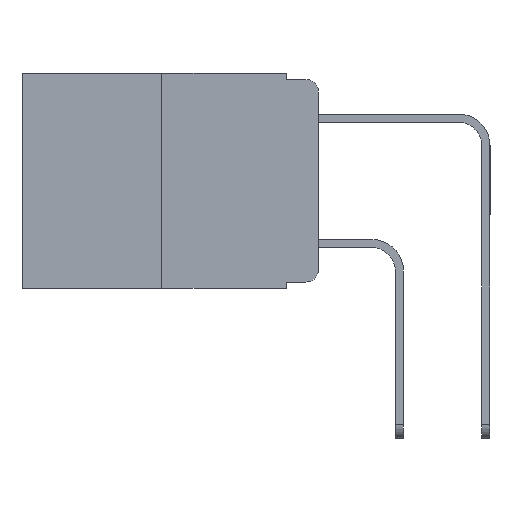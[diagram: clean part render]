
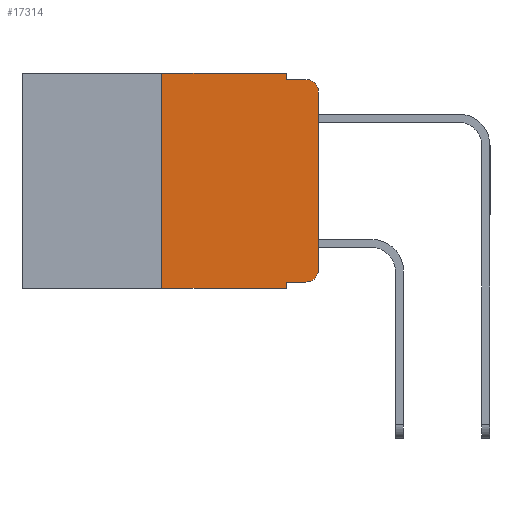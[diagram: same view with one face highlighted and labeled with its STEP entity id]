
A CAD part, left-side view. The second image highlights one B-rep face of the part: STEP entity #17314.
In plain terms, the highlighted planar face has unit normal (-1, 0, 0).
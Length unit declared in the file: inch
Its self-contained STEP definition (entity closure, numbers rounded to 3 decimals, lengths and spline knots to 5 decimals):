
#273 = ORIENTED_EDGE ( 'NONE', *, *, #997, .T. ) ;
#320 = DIRECTION ( 'NONE',  ( 1., 0., 0. ) ) ;
#418 = CARTESIAN_POINT ( 'NONE',  ( 0., 0.051, 0. ) ) ;
#564 = VECTOR ( 'NONE', #17889, 39.37008 ) ;
#701 = ORIENTED_EDGE ( 'NONE', *, *, #5124, .T. ) ;
#734 = ORIENTED_EDGE ( 'NONE', *, *, #11380, .F. ) ;
#845 = CIRCLE ( 'NONE', #16590, 0.02 ) ;
#997 = EDGE_CURVE ( 'NONE', #7784, #15619, #6264, .T. ) ;
#1246 = CARTESIAN_POINT ( 'NONE',  ( 0., 0.051, 0. ) ) ;
#1773 = VERTEX_POINT ( 'NONE', #14043 ) ;
#2390 = CARTESIAN_POINT ( 'NONE',  ( 0., 0.051, -0.01 ) ) ;
#2696 = CARTESIAN_POINT ( 'NONE',  ( 0., 0., -0.03 ) ) ;
#3437 = CARTESIAN_POINT ( 'NONE',  ( 0., 0.051, -0.333 ) ) ;
#3516 = LINE ( 'NONE', #8917, #18320 ) ;
#3554 = DIRECTION ( 'NONE',  ( 0., 0., -1. ) ) ;
#3733 = EDGE_CURVE ( 'NONE', #3890, #1773, #6423, .T. ) ;
#3751 = LINE ( 'NONE', #13107, #14830 ) ;
#3753 = VERTEX_POINT ( 'NONE', #13800 ) ;
#3842 = DIRECTION ( 'NONE',  ( -1., 0., 0. ) ) ;
#3890 = VERTEX_POINT ( 'NONE', #2390 ) ;
#4179 = LINE ( 'NONE', #12270, #564 ) ;
#4454 = ORIENTED_EDGE ( 'NONE', *, *, #13703, .T. ) ;
#4600 = CARTESIAN_POINT ( 'NONE',  ( 0., 0.051, -0.343 ) ) ;
#4791 = VECTOR ( 'NONE', #8696, 39.37008 ) ;
#5124 = EDGE_CURVE ( 'NONE', #15619, #14442, #845, .T. ) ;
#5166 = CARTESIAN_POINT ( 'NONE',  ( 0., 0.02, -0.333 ) ) ;
#5952 = EDGE_CURVE ( 'NONE', #14442, #9521, #3751, .T. ) ;
#6264 = LINE ( 'NONE', #3437, #9203 ) ;
#6355 = EDGE_CURVE ( 'NONE', #11091, #9516, #4179, .T. ) ;
#6423 = LINE ( 'NONE', #16572, #13628 ) ;
#6427 = PLANE ( 'NONE',  #10215 ) ;
#6591 = DIRECTION ( 'NONE',  ( 0., -1., 0. ) ) ;
#6727 = DIRECTION ( 'NONE',  ( -1., 0., 0. ) ) ;
#7156 = CARTESIAN_POINT ( 'NONE',  ( 0., 0.051, 0. ) ) ;
#7784 = VERTEX_POINT ( 'NONE', #11583 ) ;
#8015 = DIRECTION ( 'NONE',  ( 0., -1., 0. ) ) ;
#8182 = CARTESIAN_POINT ( 'NONE',  ( 0., 0.473, -0.343 ) ) ;
#8689 = CARTESIAN_POINT ( 'NONE',  ( 0., 0.25, 0. ) ) ;
#8696 = DIRECTION ( 'NONE',  ( 0., 0., -1. ) ) ;
#8917 = CARTESIAN_POINT ( 'NONE',  ( 0., 0.25, 0. ) ) ;
#9203 = VECTOR ( 'NONE', #6591, 39.37008 ) ;
#9336 = CARTESIAN_POINT ( 'NONE',  ( 0., 0.473, 0. ) ) ;
#9516 = VERTEX_POINT ( 'NONE', #7156 ) ;
#9521 = VERTEX_POINT ( 'NONE', #2696 ) ;
#9525 = EDGE_LOOP ( 'NONE', ( #15433, #15061, #11672, #10273, #11045, #11297, #4454, #734, #273, #701 ) ) ;
#9650 = EDGE_CURVE ( 'NONE', #3753, #11091, #3516, .T. ) ;
#10215 = AXIS2_PLACEMENT_3D ( 'NONE', #9336, #320, #10826 ) ;
#10273 = ORIENTED_EDGE ( 'NONE', *, *, #16418, .F. ) ;
#10429 = VERTEX_POINT ( 'NONE', #4600 ) ;
#10629 = VECTOR ( 'NONE', #3554, 39.37008 ) ;
#10826 = DIRECTION ( 'NONE',  ( 0., 0., -1. ) ) ;
#11045 = ORIENTED_EDGE ( 'NONE', *, *, #6355, .F. ) ;
#11091 = VERTEX_POINT ( 'NONE', #8689 ) ;
#11297 = ORIENTED_EDGE ( 'NONE', *, *, #9650, .F. ) ;
#11303 = LINE ( 'NONE', #8182, #18291 ) ;
#11380 = EDGE_CURVE ( 'NONE', #7784, #10429, #14361, .T. ) ;
#11583 = CARTESIAN_POINT ( 'NONE',  ( 0., 0.051, -0.333 ) ) ;
#11614 = CARTESIAN_POINT ( 'NONE',  ( 0., 0., -0.313 ) ) ;
#11672 = ORIENTED_EDGE ( 'NONE', *, *, #3733, .F. ) ;
#12270 = CARTESIAN_POINT ( 'NONE',  ( 0., 0.473, 0. ) ) ;
#12591 = CARTESIAN_POINT ( 'NONE',  ( 0., 0.02, -0.313 ) ) ;
#13107 = CARTESIAN_POINT ( 'NONE',  ( 0., 0., 0. ) ) ;
#13164 = CIRCLE ( 'NONE', #14956, 0.02 ) ;
#13628 = VECTOR ( 'NONE', #8015, 39.37008 ) ;
#13703 = EDGE_CURVE ( 'NONE', #3753, #10429, #11303, .T. ) ;
#13800 = CARTESIAN_POINT ( 'NONE',  ( 0., 0.25, -0.343 ) ) ;
#13955 = DIRECTION ( 'NONE',  ( 0., -1., 0. ) ) ;
#13978 = DIRECTION ( 'NONE',  ( 0., 0., -1. ) ) ;
#14043 = CARTESIAN_POINT ( 'NONE',  ( 0., 0.02, -0.01 ) ) ;
#14361 = LINE ( 'NONE', #418, #10629 ) ;
#14442 = VERTEX_POINT ( 'NONE', #11614 ) ;
#14506 = DIRECTION ( 'NONE',  ( 0., 0., 1. ) ) ;
#14830 = VECTOR ( 'NONE', #14506, 39.37008 ) ;
#14956 = AXIS2_PLACEMENT_3D ( 'NONE', #15292, #6727, #16722 ) ;
#15061 = ORIENTED_EDGE ( 'NONE', *, *, #17437, .T. ) ;
#15292 = CARTESIAN_POINT ( 'NONE',  ( 0., 0.02, -0.03 ) ) ;
#15433 = ORIENTED_EDGE ( 'NONE', *, *, #5952, .T. ) ;
#15619 = VERTEX_POINT ( 'NONE', #5166 ) ;
#16285 = LINE ( 'NONE', #1246, #4791 ) ;
#16418 = EDGE_CURVE ( 'NONE', #9516, #3890, #16285, .T. ) ;
#16572 = CARTESIAN_POINT ( 'NONE',  ( 0., 0.051, -0.01 ) ) ;
#16590 = AXIS2_PLACEMENT_3D ( 'NONE', #12591, #3842, #13978 ) ;
#16722 = DIRECTION ( 'NONE',  ( 0., 0., -1. ) ) ;
#17314 = ADVANCED_FACE ( 'NONE', ( #18609 ), #6427, .F. ) ;
#17437 = EDGE_CURVE ( 'NONE', #9521, #1773, #13164, .T. ) ;
#17889 = DIRECTION ( 'NONE',  ( 0., -1., 0. ) ) ;
#18291 = VECTOR ( 'NONE', #13955, 39.37008 ) ;
#18320 = VECTOR ( 'NONE', #18803, 39.37008 ) ;
#18609 = FACE_OUTER_BOUND ( 'NONE', #9525, .T. ) ;
#18803 = DIRECTION ( 'NONE',  ( 0., 0., 1. ) ) ;
